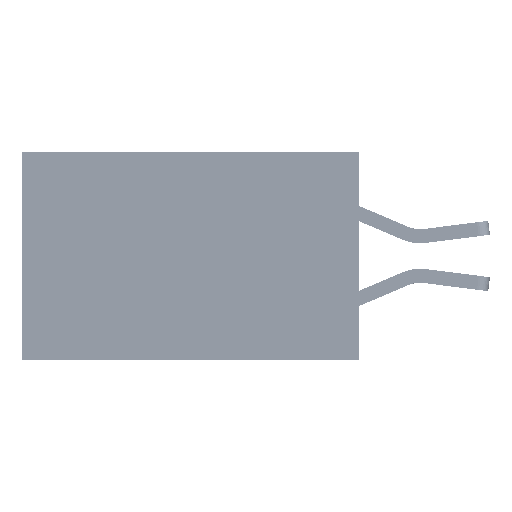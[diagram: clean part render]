
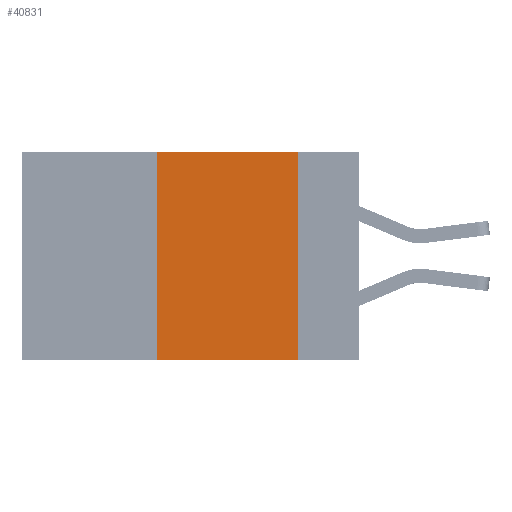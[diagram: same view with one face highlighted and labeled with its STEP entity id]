
A CAD part, left-side view. The second image highlights one B-rep face of the part: STEP entity #40831.
In plain terms, the highlighted planar face has unit normal (-1, 0, 0).
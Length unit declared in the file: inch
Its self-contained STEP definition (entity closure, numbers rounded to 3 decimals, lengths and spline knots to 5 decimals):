
#149 = AXIS2_PLACEMENT_3D ( 'NONE', #2423, #15404, #12347 ) ;
#755 = LINE ( 'NONE', #15082, #14326 ) ;
#1876 = EDGE_CURVE ( 'NONE', #19324, #22585, #14398, .T. ) ;
#2423 = CARTESIAN_POINT ( 'NONE',  ( 0., 0.6, 0. ) ) ;
#3559 = CARTESIAN_POINT ( 'NONE',  ( 0., 0.36, -0.37 ) ) ;
#3925 = DIRECTION ( 'NONE',  ( 0., 0., 1. ) ) ;
#4381 = ORIENTED_EDGE ( 'NONE', *, *, #15383, .F. ) ;
#5562 = VECTOR ( 'NONE', #10116, 39.37008 ) ;
#5569 = FACE_OUTER_BOUND ( 'NONE', #11107, .T. ) ;
#5650 = PLANE ( 'NONE',  #149 ) ;
#10116 = DIRECTION ( 'NONE',  ( 0., -1., 0. ) ) ;
#11107 = EDGE_LOOP ( 'NONE', ( #4381, #34752, #16461, #28904 ) ) ;
#11713 = CARTESIAN_POINT ( 'NONE',  ( 0., 0.6, 0. ) ) ;
#12347 = DIRECTION ( 'NONE',  ( 0., 0., -1. ) ) ;
#12770 = VERTEX_POINT ( 'NONE', #36966 ) ;
#14273 = CARTESIAN_POINT ( 'NONE',  ( 0., 0.11, 0. ) ) ;
#14326 = VECTOR ( 'NONE', #38222, 39.37008 ) ;
#14398 = LINE ( 'NONE', #29882, #5562 ) ;
#14909 = EDGE_CURVE ( 'NONE', #12770, #32975, #26926, .T. ) ;
#15082 = CARTESIAN_POINT ( 'NONE',  ( 0., 0.11, 0. ) ) ;
#15383 = EDGE_CURVE ( 'NONE', #32975, #22585, #755, .T. ) ;
#15404 = DIRECTION ( 'NONE',  ( 1., 0., 0. ) ) ;
#16461 = ORIENTED_EDGE ( 'NONE', *, *, #25789, .F. ) ;
#19324 = VERTEX_POINT ( 'NONE', #3559 ) ;
#20440 = VECTOR ( 'NONE', #3925, 39.37008 ) ;
#22585 = VERTEX_POINT ( 'NONE', #32109 ) ;
#24810 = DIRECTION ( 'NONE',  ( 0., -1., 0. ) ) ;
#25789 = EDGE_CURVE ( 'NONE', #19324, #12770, #32385, .T. ) ;
#26926 = LINE ( 'NONE', #11713, #42530 ) ;
#28904 = ORIENTED_EDGE ( 'NONE', *, *, #1876, .T. ) ;
#29882 = CARTESIAN_POINT ( 'NONE',  ( 0., 0.6, -0.37 ) ) ;
#32109 = CARTESIAN_POINT ( 'NONE',  ( 0., 0.11, -0.37 ) ) ;
#32385 = LINE ( 'NONE', #40598, #20440 ) ;
#32975 = VERTEX_POINT ( 'NONE', #14273 ) ;
#34752 = ORIENTED_EDGE ( 'NONE', *, *, #14909, .F. ) ;
#36966 = CARTESIAN_POINT ( 'NONE',  ( 0., 0.36, 0. ) ) ;
#38222 = DIRECTION ( 'NONE',  ( 0., 0., -1. ) ) ;
#40598 = CARTESIAN_POINT ( 'NONE',  ( 0., 0.36, 0. ) ) ;
#40831 = ADVANCED_FACE ( 'NONE', ( #5569 ), #5650, .F. ) ;
#42530 = VECTOR ( 'NONE', #24810, 39.37008 ) ;
